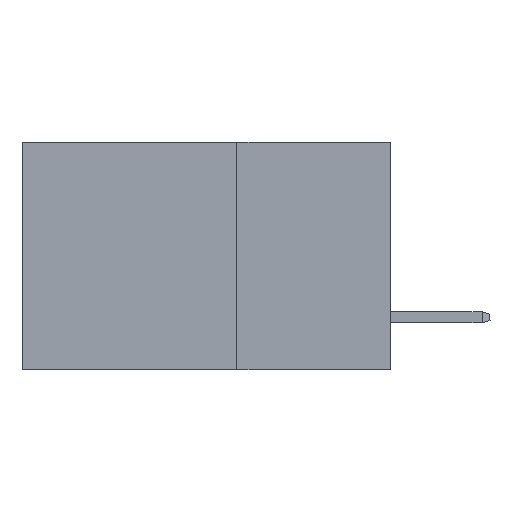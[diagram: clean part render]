
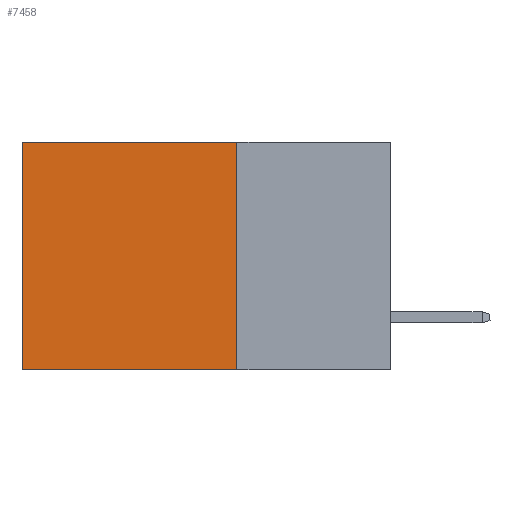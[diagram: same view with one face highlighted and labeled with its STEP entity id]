
A CAD part, left-side view. The second image highlights one B-rep face of the part: STEP entity #7458.
In plain terms, the highlighted planar face has unit normal (-1, 0, 0).
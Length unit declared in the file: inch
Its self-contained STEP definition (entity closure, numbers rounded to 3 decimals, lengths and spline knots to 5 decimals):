
#482 = VECTOR ( 'NONE', #14028, 39.37008 ) ;
#1019 = DIRECTION ( 'NONE',  ( 0., 0., -1. ) ) ;
#2105 = LINE ( 'NONE', #6655, #11148 ) ;
#2322 = EDGE_CURVE ( 'NONE', #6362, #5919, #13829, .T. ) ;
#2363 = EDGE_CURVE ( 'NONE', #15581, #6362, #3809, .T. ) ;
#3027 = ORIENTED_EDGE ( 'NONE', *, *, #12946, .T. ) ;
#3559 = CARTESIAN_POINT ( 'NONE',  ( 0.2875, 0.25, -0.37 ) ) ;
#3809 = LINE ( 'NONE', #13985, #482 ) ;
#4808 = ORIENTED_EDGE ( 'NONE', *, *, #2363, .F. ) ;
#5919 = VERTEX_POINT ( 'NONE', #12456 ) ;
#6332 = FACE_OUTER_BOUND ( 'NONE', #6798, .T. ) ;
#6362 = VERTEX_POINT ( 'NONE', #3559 ) ;
#6655 = CARTESIAN_POINT ( 'NONE',  ( 0.2875, 0.6, 0. ) ) ;
#6798 = EDGE_LOOP ( 'NONE', ( #12573, #7370, #4808, #3027 ) ) ;
#6950 = VECTOR ( 'NONE', #12500, 39.37008 ) ;
#7310 = PLANE ( 'NONE',  #9658 ) ;
#7370 = ORIENTED_EDGE ( 'NONE', *, *, #2322, .F. ) ;
#7458 = ADVANCED_FACE ( 'NONE', ( #6332 ), #7310, .F. ) ;
#8533 = DIRECTION ( 'NONE',  ( 1., 0., 0. ) ) ;
#9658 = AXIS2_PLACEMENT_3D ( 'NONE', #15398, #8533, #1019 ) ;
#10087 = VERTEX_POINT ( 'NONE', #15475 ) ;
#10255 = DIRECTION ( 'NONE',  ( 0., 0., -1. ) ) ;
#10392 = VECTOR ( 'NONE', #14853, 39.37008 ) ;
#10406 = EDGE_CURVE ( 'NONE', #10087, #5919, #2105, .T. ) ;
#10537 = LINE ( 'NONE', #11287, #6950 ) ;
#11148 = VECTOR ( 'NONE', #10255, 39.37008 ) ;
#11287 = CARTESIAN_POINT ( 'NONE',  ( 0.2875, 0.25, 0. ) ) ;
#12456 = CARTESIAN_POINT ( 'NONE',  ( 0.2875, 0.6, -0.37 ) ) ;
#12500 = DIRECTION ( 'NONE',  ( 0., 1., 0. ) ) ;
#12573 = ORIENTED_EDGE ( 'NONE', *, *, #10406, .T. ) ;
#12946 = EDGE_CURVE ( 'NONE', #15581, #10087, #10537, .T. ) ;
#13829 = LINE ( 'NONE', #14837, #10392 ) ;
#13985 = CARTESIAN_POINT ( 'NONE',  ( 0.2875, 0.25, 0. ) ) ;
#14028 = DIRECTION ( 'NONE',  ( 0., 0., -1. ) ) ;
#14837 = CARTESIAN_POINT ( 'NONE',  ( 0.2875, 0.25, -0.37 ) ) ;
#14853 = DIRECTION ( 'NONE',  ( 0., 1., 0. ) ) ;
#15387 = CARTESIAN_POINT ( 'NONE',  ( 0.2875, 0.25, 0. ) ) ;
#15398 = CARTESIAN_POINT ( 'NONE',  ( 0.2875, 0.25, 0. ) ) ;
#15475 = CARTESIAN_POINT ( 'NONE',  ( 0.2875, 0.6, 0. ) ) ;
#15581 = VERTEX_POINT ( 'NONE', #15387 ) ;
